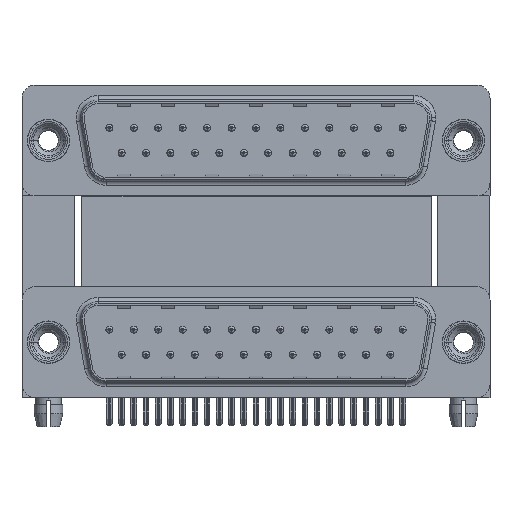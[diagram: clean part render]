
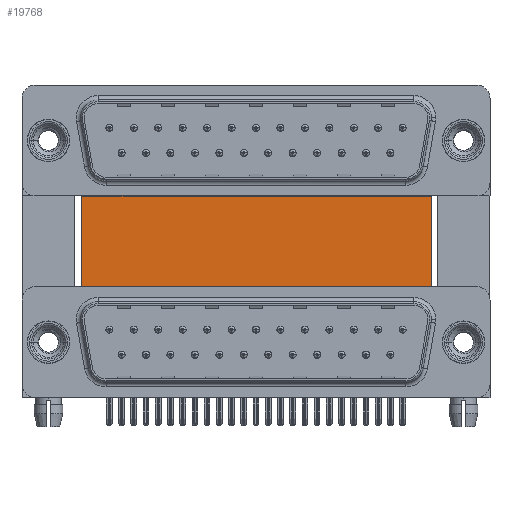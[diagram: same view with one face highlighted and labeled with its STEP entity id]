
A CAD part, top view. The second image highlights one B-rep face of the part: STEP entity #19768.
In plain terms, the highlighted planar face has unit normal (0, 0, 1).
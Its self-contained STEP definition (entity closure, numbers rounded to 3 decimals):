
#3723 = LINE ( 'NONE', #22871, #27766 ) ;
#10114 = DIRECTION ( 'NONE',  ( 1., 0., 0. ) ) ;
#11304 = VECTOR ( 'NONE', #36143, 1000. ) ;
#11537 = CARTESIAN_POINT ( 'NONE',  ( 43.43, -3.735, -12. ) ) ;
#11784 = EDGE_CURVE ( 'NONE', #27675, #22423, #17121, .T. ) ;
#13673 = EDGE_CURVE ( 'NONE', #33467, #30859, #35544, .T. ) ;
#13776 = CARTESIAN_POINT ( 'NONE',  ( 3.79, 16.585, -12. ) ) ;
#15307 = DIRECTION ( 'NONE',  ( -1., 0., 0. ) ) ;
#17121 = LINE ( 'NONE', #30133, #25873 ) ;
#17667 = CARTESIAN_POINT ( 'NONE',  ( 3.79, 16.585, -12. ) ) ;
#18083 = DIRECTION ( 'NONE',  ( 0., 0., -1. ) ) ;
#18284 = AXIS2_PLACEMENT_3D ( 'NONE', #17667, #18083, #15307 ) ;
#18933 = EDGE_CURVE ( 'NONE', #30859, #22423, #3723, .T. ) ;
#19768 = ADVANCED_FACE ( 'NONE', ( #27491 ), #40662, .F. ) ;
#21685 = EDGE_LOOP ( 'NONE', ( #36210, #35599, #23275, #24775 ) ) ;
#22423 = VERTEX_POINT ( 'NONE', #11537 ) ;
#22871 = CARTESIAN_POINT ( 'NONE',  ( 43.43, 16.585, -12. ) ) ;
#23275 = ORIENTED_EDGE ( 'NONE', *, *, #13673, .F. ) ;
#24775 = ORIENTED_EDGE ( 'NONE', *, *, #36858, .T. ) ;
#24957 = VECTOR ( 'NONE', #35115, 1000. ) ;
#25873 = VECTOR ( 'NONE', #10114, 1000. ) ;
#27491 = FACE_OUTER_BOUND ( 'NONE', #21685, .T. ) ;
#27675 = VERTEX_POINT ( 'NONE', #34190 ) ;
#27766 = VECTOR ( 'NONE', #41816, 1000. ) ;
#29370 = CARTESIAN_POINT ( 'NONE',  ( 3.79, 16.585, -12. ) ) ;
#30133 = CARTESIAN_POINT ( 'NONE',  ( 3.79, -3.735, -12. ) ) ;
#30135 = CARTESIAN_POINT ( 'NONE',  ( 43.43, 16.585, -12. ) ) ;
#30859 = VERTEX_POINT ( 'NONE', #30135 ) ;
#33467 = VERTEX_POINT ( 'NONE', #39138 ) ;
#34190 = CARTESIAN_POINT ( 'NONE',  ( 3.79, -3.735, -12. ) ) ;
#35115 = DIRECTION ( 'NONE',  ( 1., 0., 0. ) ) ;
#35544 = LINE ( 'NONE', #29370, #24957 ) ;
#35599 = ORIENTED_EDGE ( 'NONE', *, *, #18933, .F. ) ;
#36143 = DIRECTION ( 'NONE',  ( 0., -1., 0. ) ) ;
#36210 = ORIENTED_EDGE ( 'NONE', *, *, #11784, .T. ) ;
#36858 = EDGE_CURVE ( 'NONE', #33467, #27675, #39755, .T. ) ;
#39138 = CARTESIAN_POINT ( 'NONE',  ( 3.79, 16.585, -12. ) ) ;
#39755 = LINE ( 'NONE', #13776, #11304 ) ;
#40662 = PLANE ( 'NONE',  #18284 ) ;
#41816 = DIRECTION ( 'NONE',  ( 0., -1., 0. ) ) ;
